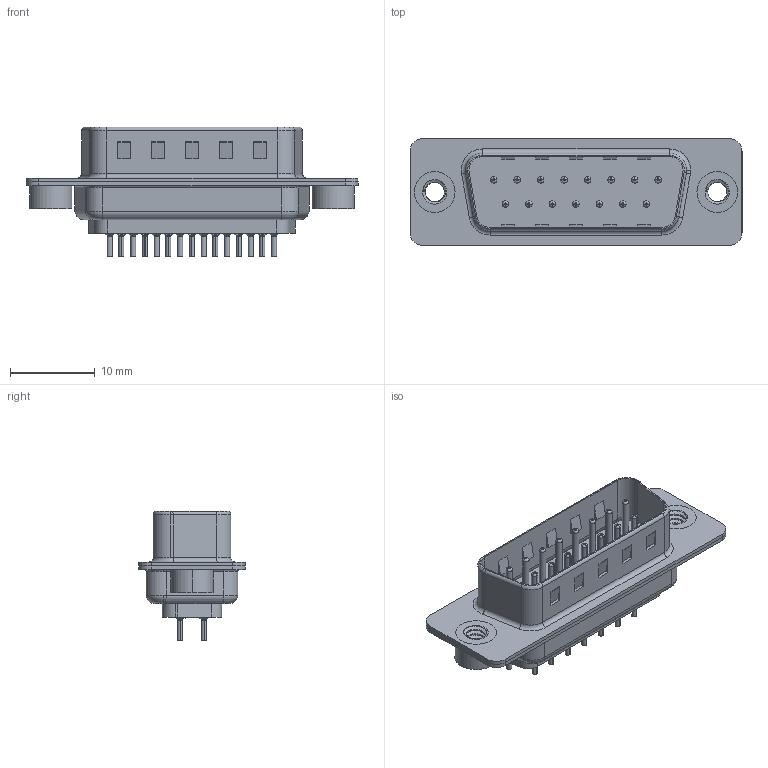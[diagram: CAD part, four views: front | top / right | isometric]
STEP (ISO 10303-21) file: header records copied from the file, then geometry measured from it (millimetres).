
FILE_DESCRIPTION (( 'STEP AP203' ), '1' );
FILE_NAME ('627-015-228-542.STEP', '2018-10-04T03:28:42', ( '' ), ( '' ), 'SwSTEP 2.0', 'SolidWorks 2016', '' );
FILE_SCHEMA (( 'CONFIG_CONTROL_DESIGN' ));
Length unit declared in the file: millimetre
Products named in the file (7): 627 Housing_15 LP; 627 Shell Front_15 Contacts; 627 Shell Rear_15 Contacts; 627 Contact Row 1_28L; 627 Contact Row 2_28L; 627 4-40 Threaded Rivet; 627-015-228-542
Assembly tree (20 placements, depth 2):
  627-015-228-542
    627 Housing_15 LP
    627 Shell Front_15 Contacts
    627 Shell Rear_15 Contacts
    627 Contact Row 1_28L  x8
    627 Contact Row 2_28L  x7
    627 4-40 Threaded Rivet  x2
Bounding box: 39.15 x 12.6 x 15.3 mm (x, y, z)
Volume: 1825.5 mm3; surface area: 5312.3 mm2
Topology: 20 solids, 20 shells, 1810 faces, 4714 edges, 2925 vertices
Faces by surface type: cylinder 688, plane 499, torus 461, cone 156, bspline 6
Entity records: 21370 total; most frequent: CARTESIAN_POINT 5214, DIRECTION 3365, ORIENTED_EDGE 3034, EDGE_CURVE 1517, AXIS2_PLACEMENT_3D 1334, VERTEX_POINT 961, EDGE_LOOP 710, CIRCLE 707
